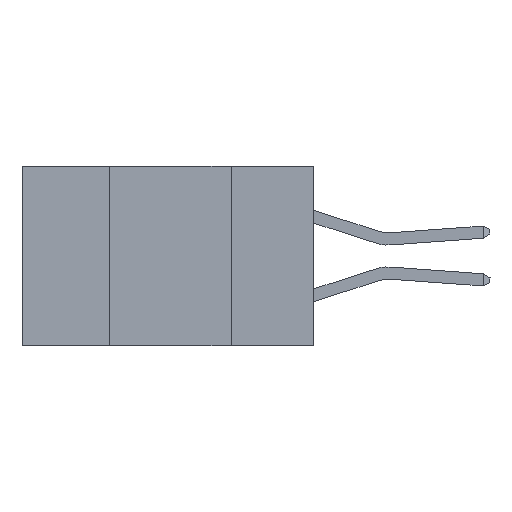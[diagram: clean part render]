
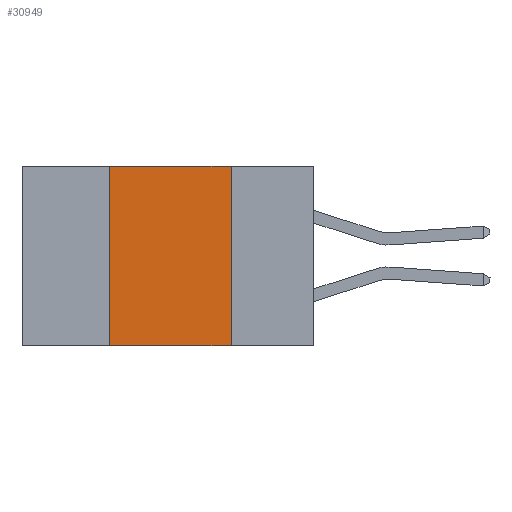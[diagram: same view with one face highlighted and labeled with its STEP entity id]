
A CAD part, left-side view. The second image highlights one B-rep face of the part: STEP entity #30949.
In plain terms, the highlighted planar face has unit normal (-1, 0, 0).
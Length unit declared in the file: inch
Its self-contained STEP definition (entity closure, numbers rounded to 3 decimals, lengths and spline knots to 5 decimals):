
#23 = DIRECTION ( 'NONE',  ( 0., 0., -1. ) ) ;
#225 = DIRECTION ( 'NONE',  ( 1., 0., 0. ) ) ;
#584 = PLANE ( 'NONE',  #34804 ) ;
#1795 = VERTEX_POINT ( 'NONE', #21424 ) ;
#4454 = LINE ( 'NONE', #10272, #5035 ) ;
#4646 = CARTESIAN_POINT ( 'NONE',  ( 0., 0.42, -0.37 ) ) ;
#4830 = DIRECTION ( 'NONE',  ( 0., 0., -1. ) ) ;
#5035 = VECTOR ( 'NONE', #13162, 39.37008 ) ;
#5613 = EDGE_CURVE ( 'NONE', #32817, #11526, #22985, .T. ) ;
#8701 = CARTESIAN_POINT ( 'NONE',  ( 0., 0.17, 0. ) ) ;
#9082 = VERTEX_POINT ( 'NONE', #4646 ) ;
#9306 = VECTOR ( 'NONE', #4830, 39.37008 ) ;
#10056 = CARTESIAN_POINT ( 'NONE',  ( 0., 0.6, -0.37 ) ) ;
#10272 = CARTESIAN_POINT ( 'NONE',  ( 0., 0.6, 0. ) ) ;
#10729 = ORIENTED_EDGE ( 'NONE', *, *, #30916, .F. ) ;
#11269 = LINE ( 'NONE', #23039, #34197 ) ;
#11526 = VERTEX_POINT ( 'NONE', #31210 ) ;
#13162 = DIRECTION ( 'NONE',  ( 0., -1., 0. ) ) ;
#14141 = ORIENTED_EDGE ( 'NONE', *, *, #28467, .F. ) ;
#14529 = EDGE_LOOP ( 'NONE', ( #36399, #14141, #10729, #31813 ) ) ;
#21424 = CARTESIAN_POINT ( 'NONE',  ( 0., 0.42, 0. ) ) ;
#22210 = LINE ( 'NONE', #10056, #33345 ) ;
#22985 = LINE ( 'NONE', #34388, #9306 ) ;
#22996 = EDGE_CURVE ( 'NONE', #9082, #11526, #22210, .T. ) ;
#23039 = CARTESIAN_POINT ( 'NONE',  ( 0., 0.42, 0. ) ) ;
#28467 = EDGE_CURVE ( 'NONE', #1795, #32817, #4454, .T. ) ;
#30539 = DIRECTION ( 'NONE',  ( 0., -1., 0. ) ) ;
#30916 = EDGE_CURVE ( 'NONE', #9082, #1795, #11269, .T. ) ;
#30949 = ADVANCED_FACE ( 'NONE', ( #38099 ), #584, .F. ) ;
#31210 = CARTESIAN_POINT ( 'NONE',  ( 0., 0.17, -0.37 ) ) ;
#31813 = ORIENTED_EDGE ( 'NONE', *, *, #22996, .T. ) ;
#32486 = CARTESIAN_POINT ( 'NONE',  ( 0., 0.6, 0. ) ) ;
#32817 = VERTEX_POINT ( 'NONE', #8701 ) ;
#33345 = VECTOR ( 'NONE', #30539, 39.37008 ) ;
#34197 = VECTOR ( 'NONE', #34825, 39.37008 ) ;
#34388 = CARTESIAN_POINT ( 'NONE',  ( 0., 0.17, 0. ) ) ;
#34804 = AXIS2_PLACEMENT_3D ( 'NONE', #32486, #225, #23 ) ;
#34825 = DIRECTION ( 'NONE',  ( 0., 0., 1. ) ) ;
#36399 = ORIENTED_EDGE ( 'NONE', *, *, #5613, .F. ) ;
#38099 = FACE_OUTER_BOUND ( 'NONE', #14529, .T. ) ;
